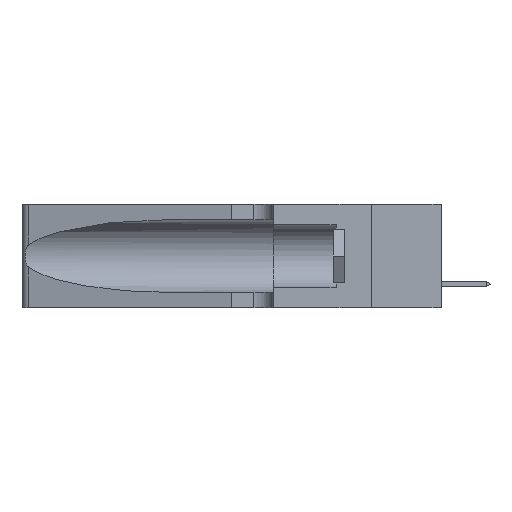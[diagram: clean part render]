
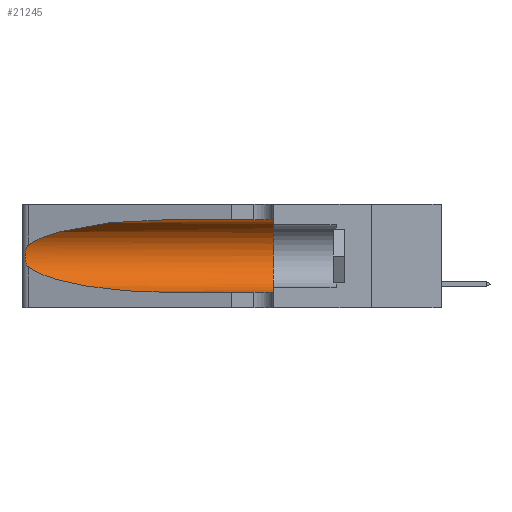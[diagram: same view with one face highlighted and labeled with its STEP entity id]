
A CAD part, left-side view. The second image highlights one B-rep face of the part: STEP entity #21245.
In plain terms, the highlighted cylindrical face has radius 3.308 mm (diameter 6.617 mm), a partial arc.
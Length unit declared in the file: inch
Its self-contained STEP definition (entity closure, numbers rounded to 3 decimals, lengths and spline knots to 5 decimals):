
#479 = DIRECTION ( 'NONE',  ( 0., 1., 0. ) ) ;
#744 =( BOUNDED_CURVE ( )  B_SPLINE_CURVE ( 3, ( #11447, #2709, #4486, #20318 ),
 .UNSPECIFIED., .F., .T. ) 
 B_SPLINE_CURVE_WITH_KNOTS ( ( 4, 4 ),
 ( 3.44316, 4.71239 ),
 .UNSPECIFIED. ) 
 CURVE ( )  GEOMETRIC_REPRESENTATION_ITEM ( )  RATIONAL_B_SPLINE_CURVE ( ( 1., 0.87, 0.87, 1. ) ) 
 REPRESENTATION_ITEM ( '' )  );
#1031 = CARTESIAN_POINT ( 'NONE',  ( 0.1305, 0.35, 0.31525 ) ) ;
#1302 = CARTESIAN_POINT ( 'NONE',  ( 0.25856, 1.23593, 0.16098 ) ) ;
#1326 = CARTESIAN_POINT ( 'NONE',  ( 0.1305, 0.35, 0.05475 ) ) ;
#2433 = DIRECTION ( 'NONE',  ( 0., -1., 0. ) ) ;
#2709 = CARTESIAN_POINT ( 'NONE',  ( 0.2373, 1.15595, 0.08982 ) ) ;
#2774 = AXIS2_PLACEMENT_3D ( 'NONE', #21562, #479, #12777 ) ;
#3160 = CARTESIAN_POINT ( 'NONE',  ( 0.25555, 1.22993, 0.14849 ) ) ;
#3668 = VERTEX_POINT ( 'NONE', #11807 ) ;
#3969 = VERTEX_POINT ( 'NONE', #18872 ) ;
#4087 = CYLINDRICAL_SURFACE ( 'NONE', #17753, 0.13025 ) ;
#4222 = EDGE_CURVE ( 'NONE', #3668, #20039, #13557, .T. ) ;
#4486 = CARTESIAN_POINT ( 'NONE',  ( 0.18966, 0.96281, 0.05475 ) ) ;
#4690 = CARTESIAN_POINT ( 'NONE',  ( 0.25787, 1.23484, 0.2124 ) ) ;
#5211 = FACE_OUTER_BOUND ( 'NONE', #13875, .T. ) ;
#5815 = CARTESIAN_POINT ( 'NONE',  ( 0.1305, 1.61858, 0.05475 ) ) ;
#6613 = ORIENTED_EDGE ( 'NONE', *, *, #12454, .T. ) ;
#6706 = DIRECTION ( 'NONE',  ( 0., -1., 0. ) ) ;
#6755 = EDGE_CURVE ( 'NONE', #17772, #3668, #744, .T. ) ;
#7514 = EDGE_CURVE ( 'NONE', #12995, #20039, #17303, .T. ) ;
#7699 = CARTESIAN_POINT ( 'NONE',  ( 0.25487, 1.22718, 0.22369 ) ) ;
#7821 = CARTESIAN_POINT ( 'NONE',  ( 0.1305, 0.72297, 0.31525 ) ) ;
#8826 = ORIENTED_EDGE ( 'NONE', *, *, #16327, .F. ) ;
#9304 = VECTOR ( 'NONE', #6706, 39.37008 ) ;
#9413 = VECTOR ( 'NONE', #2433, 39.37008 ) ;
#9422 = ORIENTED_EDGE ( 'NONE', *, *, #13477, .T. ) ;
#10872 = CARTESIAN_POINT ( 'NONE',  ( 0.25487, 1.22718, 0.14631 ) ) ;
#11447 = CARTESIAN_POINT ( 'NONE',  ( 0.25487, 1.22718, 0.14631 ) ) ;
#11807 = CARTESIAN_POINT ( 'NONE',  ( 0.1305, 0.72297, 0.05475 ) ) ;
#12454 = EDGE_CURVE ( 'NONE', #19266, #3969, #21599, .T. ) ;
#12582 = CARTESIAN_POINT ( 'NONE',  ( 0.25487, 1.22718, 0.22369 ) ) ;
#12777 = DIRECTION ( 'NONE',  ( 0., 0., 1. ) ) ;
#12995 = VERTEX_POINT ( 'NONE', #1031 ) ;
#13276 = CARTESIAN_POINT ( 'NONE',  ( 0.26075, 1.23896, 0.19203 ) ) ;
#13356 = CARTESIAN_POINT ( 'NONE',  ( 0.25639, 1.23184, 0.21858 ) ) ;
#13477 = EDGE_CURVE ( 'NONE', #3969, #17772, #17566, .T. ) ;
#13557 = LINE ( 'NONE', #5815, #9413 ) ;
#13678 = CARTESIAN_POINT ( 'NONE',  ( 0.25639, 1.23186, 0.15144 ) ) ;
#13875 = EDGE_LOOP ( 'NONE', ( #6613, #9422, #22651, #19893, #14929, #8826 ) ) ;
#14283 = CARTESIAN_POINT ( 'NONE',  ( 0.2373, 1.15595, 0.28018 ) ) ;
#14363 = CARTESIAN_POINT ( 'NONE',  ( 0.18966, 0.96281, 0.31525 ) ) ;
#14799 = LINE ( 'NONE', #15444, #9304 ) ;
#14929 = ORIENTED_EDGE ( 'NONE', *, *, #7514, .F. ) ;
#15044 = CARTESIAN_POINT ( 'NONE',  ( 0.25789, 1.23486, 0.15765 ) ) ;
#15203 = CARTESIAN_POINT ( 'NONE',  ( 0.25555, 1.22994, 0.2215 ) ) ;
#15366 = CARTESIAN_POINT ( 'NONE',  ( 0.26017, 1.23833, 0.17102 ) ) ;
#15444 = CARTESIAN_POINT ( 'NONE',  ( 0.1305, 1.61858, 0.31525 ) ) ;
#15864 = DIRECTION ( 'NONE',  ( 0., -1., 0. ) ) ;
#16327 = EDGE_CURVE ( 'NONE', #19266, #12995, #14799, .T. ) ;
#17303 = CIRCLE ( 'NONE', #2774, 0.13025 ) ;
#17456 = CARTESIAN_POINT ( 'NONE',  ( 0.1305, 1.61858, 0.185 ) ) ;
#17566 = B_SPLINE_CURVE_WITH_KNOTS ( 'NONE', 3,
 ( #7699, #15203, #13356, #4690, #18770, #20621, #13276, #20697, #15366, #1302, #15044, #13678, #3160, #19154 ),
 .UNSPECIFIED., .F., .F.,
 ( 4, 2, 2, 2, 2, 2, 4 ),
 ( 0., 0.00027, 0.00053, 0.00107, 0.0016, 0.00187, 0.00214 ),
 .UNSPECIFIED. ) ;
#17753 = AXIS2_PLACEMENT_3D ( 'NONE', #17456, #15864, #19416 ) ;
#17772 = VERTEX_POINT ( 'NONE', #10872 ) ;
#18770 = CARTESIAN_POINT ( 'NONE',  ( 0.25854, 1.2359, 0.20912 ) ) ;
#18872 = CARTESIAN_POINT ( 'NONE',  ( 0.25487, 1.22718, 0.22369 ) ) ;
#19154 = CARTESIAN_POINT ( 'NONE',  ( 0.25487, 1.22718, 0.14631 ) ) ;
#19266 = VERTEX_POINT ( 'NONE', #7821 ) ;
#19416 = DIRECTION ( 'NONE',  ( 0., 0., -1. ) ) ;
#19767 = CARTESIAN_POINT ( 'NONE',  ( 0.1305, 0.72297, 0.31525 ) ) ;
#19893 = ORIENTED_EDGE ( 'NONE', *, *, #4222, .T. ) ;
#20039 = VERTEX_POINT ( 'NONE', #1326 ) ;
#20318 = CARTESIAN_POINT ( 'NONE',  ( 0.1305, 0.72297, 0.05475 ) ) ;
#20621 = CARTESIAN_POINT ( 'NONE',  ( 0.26018, 1.23835, 0.19895 ) ) ;
#20697 = CARTESIAN_POINT ( 'NONE',  ( 0.26075, 1.23896, 0.178 ) ) ;
#21245 = ADVANCED_FACE ( 'NONE', ( #5211 ), #4087, .F. ) ;
#21562 = CARTESIAN_POINT ( 'NONE',  ( 0.1305, 0.35, 0.185 ) ) ;
#21599 =( BOUNDED_CURVE ( )  B_SPLINE_CURVE ( 3, ( #19767, #14363, #14283, #12582 ),
 .UNSPECIFIED., .F., .F. ) 
 B_SPLINE_CURVE_WITH_KNOTS ( ( 4, 4 ),
 ( 1.5708, 2.84003 ),
 .UNSPECIFIED. ) 
 CURVE ( )  GEOMETRIC_REPRESENTATION_ITEM ( )  RATIONAL_B_SPLINE_CURVE ( ( 1., 0.87, 0.87, 1. ) ) 
 REPRESENTATION_ITEM ( '' )  );
#22651 = ORIENTED_EDGE ( 'NONE', *, *, #6755, .T. ) ;
